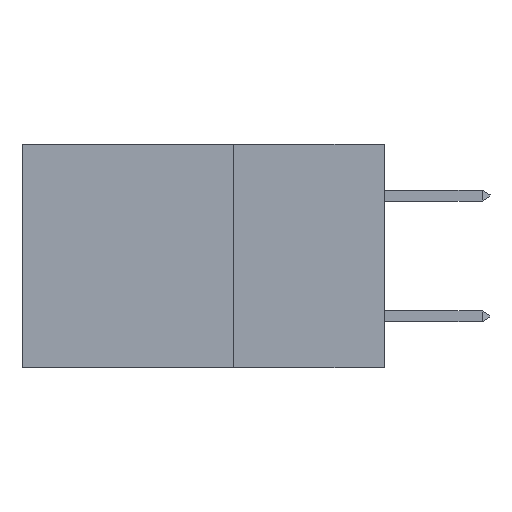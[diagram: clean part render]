
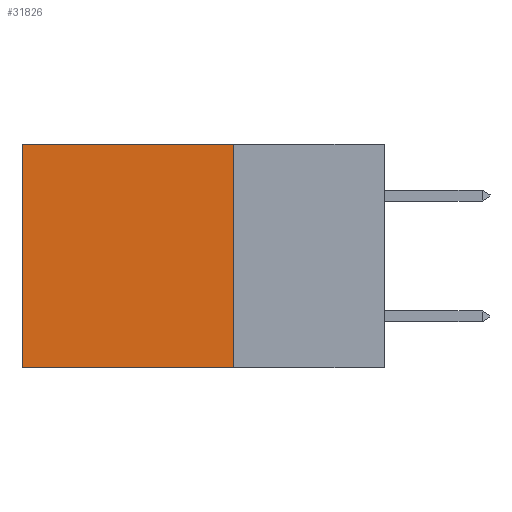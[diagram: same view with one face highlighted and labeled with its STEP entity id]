
A CAD part, left-side view. The second image highlights one B-rep face of the part: STEP entity #31826.
In plain terms, the highlighted planar face has unit normal (-1, 0, 0).
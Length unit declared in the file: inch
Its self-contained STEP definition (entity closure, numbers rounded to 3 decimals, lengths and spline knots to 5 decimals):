
#406 = VERTEX_POINT ( 'NONE', #10701 ) ;
#709 = LINE ( 'NONE', #24679, #29737 ) ;
#1673 = EDGE_CURVE ( 'NONE', #12329, #9886, #28826, .T. ) ;
#3918 = CARTESIAN_POINT ( 'NONE',  ( 0.2875, 0.6, -0.37 ) ) ;
#3986 = AXIS2_PLACEMENT_3D ( 'NONE', #23254, #9405, #28780 ) ;
#4953 = LINE ( 'NONE', #10160, #34488 ) ;
#6008 = VECTOR ( 'NONE', #15420, 39.37008 ) ;
#6505 = PLANE ( 'NONE',  #3986 ) ;
#6613 = VECTOR ( 'NONE', #17519, 39.37008 ) ;
#9405 = DIRECTION ( 'NONE',  ( 1., 0., 0. ) ) ;
#9886 = VERTEX_POINT ( 'NONE', #3918 ) ;
#10089 = CARTESIAN_POINT ( 'NONE',  ( 0.2875, 0.25, -0.37 ) ) ;
#10160 = CARTESIAN_POINT ( 'NONE',  ( 0.2875, 0.25, 0. ) ) ;
#10701 = CARTESIAN_POINT ( 'NONE',  ( 0.2875, 0.25, 0. ) ) ;
#12329 = VERTEX_POINT ( 'NONE', #10089 ) ;
#13089 = ORIENTED_EDGE ( 'NONE', *, *, #1673, .F. ) ;
#13511 = EDGE_CURVE ( 'NONE', #20594, #9886, #26515, .T. ) ;
#14772 = CARTESIAN_POINT ( 'NONE',  ( 0.2875, 0.25, -0.37 ) ) ;
#15420 = DIRECTION ( 'NONE',  ( 0., 0., -1. ) ) ;
#17519 = DIRECTION ( 'NONE',  ( 0., 1., 0. ) ) ;
#20594 = VERTEX_POINT ( 'NONE', #34851 ) ;
#20980 = CARTESIAN_POINT ( 'NONE',  ( 0.2875, 0.6, 0. ) ) ;
#21205 = DIRECTION ( 'NONE',  ( 0., 0., -1. ) ) ;
#22685 = EDGE_CURVE ( 'NONE', #406, #20594, #709, .T. ) ;
#23254 = CARTESIAN_POINT ( 'NONE',  ( 0.2875, 0.25, 0. ) ) ;
#24679 = CARTESIAN_POINT ( 'NONE',  ( 0.2875, 0.25, 0. ) ) ;
#24868 = ORIENTED_EDGE ( 'NONE', *, *, #13511, .T. ) ;
#26515 = LINE ( 'NONE', #20980, #6008 ) ;
#27768 = FACE_OUTER_BOUND ( 'NONE', #33178, .T. ) ;
#28780 = DIRECTION ( 'NONE',  ( 0., 0., -1. ) ) ;
#28826 = LINE ( 'NONE', #14772, #6613 ) ;
#29690 = ORIENTED_EDGE ( 'NONE', *, *, #22685, .T. ) ;
#29737 = VECTOR ( 'NONE', #32834, 39.37008 ) ;
#31826 = ADVANCED_FACE ( 'NONE', ( #27768 ), #6505, .F. ) ;
#32834 = DIRECTION ( 'NONE',  ( 0., 1., 0. ) ) ;
#33178 = EDGE_LOOP ( 'NONE', ( #24868, #13089, #34666, #29690 ) ) ;
#33421 = EDGE_CURVE ( 'NONE', #406, #12329, #4953, .T. ) ;
#34488 = VECTOR ( 'NONE', #21205, 39.37008 ) ;
#34666 = ORIENTED_EDGE ( 'NONE', *, *, #33421, .F. ) ;
#34851 = CARTESIAN_POINT ( 'NONE',  ( 0.2875, 0.6, 0. ) ) ;
